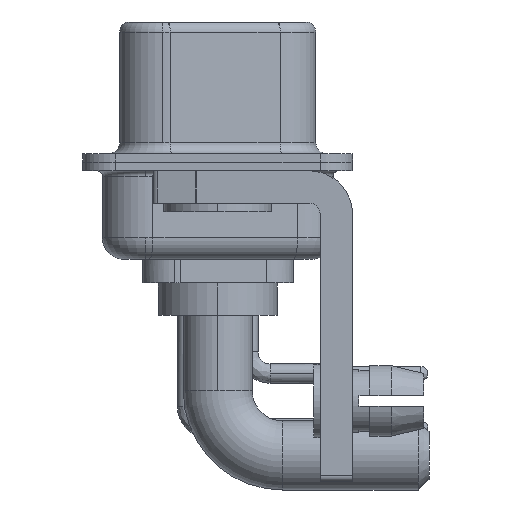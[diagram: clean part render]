
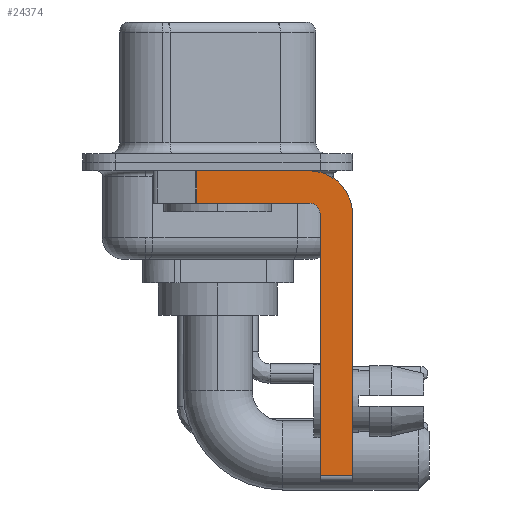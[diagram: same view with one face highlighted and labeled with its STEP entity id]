
A CAD part, left-side view. The second image highlights one B-rep face of the part: STEP entity #24374.
In plain terms, the highlighted planar face has unit normal (-1, 0, 0).
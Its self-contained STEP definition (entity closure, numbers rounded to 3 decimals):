
#220 = ORIENTED_EDGE ( 'NONE', *, *, #28409, .F. ) ;
#810 = CARTESIAN_POINT ( 'NONE',  ( -2.9, -4.25, -2.4 ) ) ;
#891 = CARTESIAN_POINT ( 'NONE',  ( -2.9, 0.978, -1.9 ) ) ;
#1488 = VERTEX_POINT ( 'NONE', #891 ) ;
#1781 = CARTESIAN_POINT ( 'NONE',  ( -2.9, -4.25, -1.9 ) ) ;
#2296 = EDGE_LOOP ( 'NONE', ( #220, #7860, #19373, #23999, #4862, #28705, #16245, #28285 ) ) ;
#3200 = VERTEX_POINT ( 'NONE', #29447 ) ;
#3207 = VECTOR ( 'NONE', #22636, 1000. ) ;
#3834 = DIRECTION ( 'NONE',  ( 0., 0., -1. ) ) ;
#4681 = VERTEX_POINT ( 'NONE', #7345 ) ;
#4756 = VECTOR ( 'NONE', #7383, 1000. ) ;
#4862 = ORIENTED_EDGE ( 'NONE', *, *, #17629, .F. ) ;
#5077 = CARTESIAN_POINT ( 'NONE',  ( -2.9, -6.25, -2.4 ) ) ;
#5546 = CARTESIAN_POINT ( 'NONE',  ( -2.9, -6.25, -14.55 ) ) ;
#6180 = DIRECTION ( 'NONE',  ( 0., -1., 0. ) ) ;
#7345 = CARTESIAN_POINT ( 'NONE',  ( -2.9, 0.978, -0.4 ) ) ;
#7383 = DIRECTION ( 'NONE',  ( 0., 1., 0. ) ) ;
#7533 = EDGE_CURVE ( 'NONE', #4681, #1488, #22800, .T. ) ;
#7641 = VECTOR ( 'NONE', #6180, 1000. ) ;
#7847 = DIRECTION ( 'NONE',  ( 0., 0., -1. ) ) ;
#7860 = ORIENTED_EDGE ( 'NONE', *, *, #7533, .T. ) ;
#8069 = CIRCLE ( 'NONE', #17869, 2. ) ;
#8383 = VECTOR ( 'NONE', #15431, 1000. ) ;
#8408 = CARTESIAN_POINT ( 'NONE',  ( -2.9, -4.75, -14.55 ) ) ;
#9310 = DIRECTION ( 'NONE',  ( 0., 0., 1. ) ) ;
#10523 = CARTESIAN_POINT ( 'NONE',  ( -2.9, 0.978, -1.9 ) ) ;
#11652 = CARTESIAN_POINT ( 'NONE',  ( -2.9, 3., -0.4 ) ) ;
#11714 = EDGE_CURVE ( 'NONE', #22380, #29342, #15137, .T. ) ;
#11956 = LINE ( 'NONE', #11652, #20941 ) ;
#12246 = VERTEX_POINT ( 'NONE', #1781 ) ;
#12396 = AXIS2_PLACEMENT_3D ( 'NONE', #23742, #28041, #9310 ) ;
#15074 = EDGE_CURVE ( 'NONE', #24811, #12246, #25631, .T. ) ;
#15137 = LINE ( 'NONE', #25274, #19444 ) ;
#15431 = DIRECTION ( 'NONE',  ( 0., 0., -1. ) ) ;
#16040 = LINE ( 'NONE', #27550, #3207 ) ;
#16245 = ORIENTED_EDGE ( 'NONE', *, *, #11714, .F. ) ;
#17629 = EDGE_CURVE ( 'NONE', #21300, #24811, #16040, .T. ) ;
#17782 = PLANE ( 'NONE',  #20008 ) ;
#17869 = AXIS2_PLACEMENT_3D ( 'NONE', #810, #26430, #7847 ) ;
#18313 = EDGE_CURVE ( 'NONE', #3200, #22380, #8069, .T. ) ;
#19016 = DIRECTION ( 'NONE',  ( 0., -1., 0. ) ) ;
#19373 = ORIENTED_EDGE ( 'NONE', *, *, #28011, .F. ) ;
#19444 = VECTOR ( 'NONE', #24957, 1000. ) ;
#20008 = AXIS2_PLACEMENT_3D ( 'NONE', #27144, #20230, #3834 ) ;
#20230 = DIRECTION ( 'NONE',  ( 1., 0., 0. ) ) ;
#20941 = VECTOR ( 'NONE', #19016, 1000. ) ;
#21300 = VERTEX_POINT ( 'NONE', #8408 ) ;
#22380 = VERTEX_POINT ( 'NONE', #5077 ) ;
#22636 = DIRECTION ( 'NONE',  ( 0., 0., 1. ) ) ;
#22800 = LINE ( 'NONE', #10523, #8383 ) ;
#23742 = CARTESIAN_POINT ( 'NONE',  ( -2.9, -4.25, -2.4 ) ) ;
#23807 = LINE ( 'NONE', #25970, #4756 ) ;
#23999 = ORIENTED_EDGE ( 'NONE', *, *, #15074, .F. ) ;
#24374 = ADVANCED_FACE ( 'NONE', ( #26698 ), #17782, .F. ) ;
#24811 = VERTEX_POINT ( 'NONE', #27986 ) ;
#24957 = DIRECTION ( 'NONE',  ( 0., 0., -1. ) ) ;
#25274 = CARTESIAN_POINT ( 'NONE',  ( -2.9, -6.25, -2.4 ) ) ;
#25631 = CIRCLE ( 'NONE', #12396, 0.5 ) ;
#25685 = EDGE_CURVE ( 'NONE', #21300, #29342, #27359, .T. ) ;
#25970 = CARTESIAN_POINT ( 'NONE',  ( -2.9, -4.25, -1.9 ) ) ;
#26430 = DIRECTION ( 'NONE',  ( 1., 0., 0. ) ) ;
#26698 = FACE_OUTER_BOUND ( 'NONE', #2296, .T. ) ;
#27144 = CARTESIAN_POINT ( 'NONE',  ( -2.9, -4.25, -2.4 ) ) ;
#27359 = LINE ( 'NONE', #27662, #7641 ) ;
#27550 = CARTESIAN_POINT ( 'NONE',  ( -2.9, -4.75, -14.8 ) ) ;
#27662 = CARTESIAN_POINT ( 'NONE',  ( -2.9, -4.25, -14.55 ) ) ;
#27986 = CARTESIAN_POINT ( 'NONE',  ( -2.9, -4.75, -2.4 ) ) ;
#28011 = EDGE_CURVE ( 'NONE', #12246, #1488, #23807, .T. ) ;
#28041 = DIRECTION ( 'NONE',  ( -1., 0., 0. ) ) ;
#28285 = ORIENTED_EDGE ( 'NONE', *, *, #18313, .F. ) ;
#28409 = EDGE_CURVE ( 'NONE', #4681, #3200, #11956, .T. ) ;
#28705 = ORIENTED_EDGE ( 'NONE', *, *, #25685, .T. ) ;
#29342 = VERTEX_POINT ( 'NONE', #5546 ) ;
#29447 = CARTESIAN_POINT ( 'NONE',  ( -2.9, -4.25, -0.4 ) ) ;
